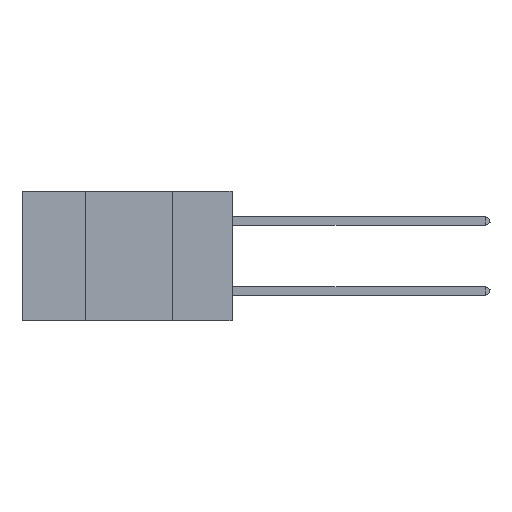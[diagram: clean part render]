
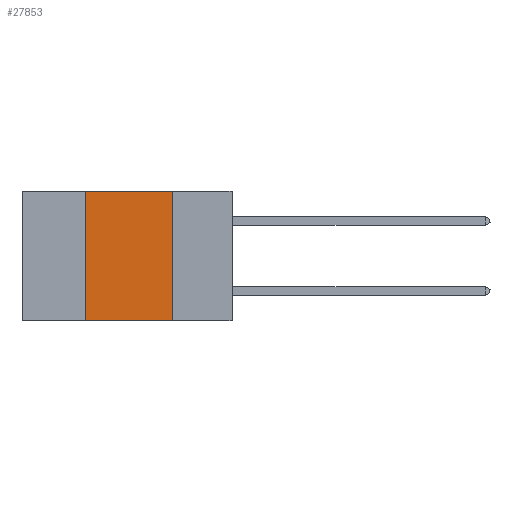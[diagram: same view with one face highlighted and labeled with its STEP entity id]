
A CAD part, left-side view. The second image highlights one B-rep face of the part: STEP entity #27853.
In plain terms, the highlighted planar face has unit normal (-1, 0, 0).
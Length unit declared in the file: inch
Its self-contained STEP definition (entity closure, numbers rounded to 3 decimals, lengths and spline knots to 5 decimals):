
#688 = LINE ( 'NONE', #7129, #45651 ) ;
#830 = DIRECTION ( 'NONE',  ( 0., 0., -1. ) ) ;
#3202 = CARTESIAN_POINT ( 'NONE',  ( 0., 0.6, -0.37 ) ) ;
#3788 = LINE ( 'NONE', #24163, #15774 ) ;
#3945 = DIRECTION ( 'NONE',  ( 0., -1., 0. ) ) ;
#5041 = DIRECTION ( 'NONE',  ( 0., -1., 0. ) ) ;
#7129 = CARTESIAN_POINT ( 'NONE',  ( 0., 0.6, 0. ) ) ;
#8610 = EDGE_CURVE ( 'NONE', #33433, #15304, #44343, .T. ) ;
#11123 = ORIENTED_EDGE ( 'NONE', *, *, #41493, .F. ) ;
#15304 = VERTEX_POINT ( 'NONE', #42648 ) ;
#15774 = VECTOR ( 'NONE', #830, 39.37008 ) ;
#16194 = CARTESIAN_POINT ( 'NONE',  ( 0., 0.6, 0. ) ) ;
#17471 = VECTOR ( 'NONE', #45445, 39.37008 ) ;
#20066 = PLANE ( 'NONE',  #45449 ) ;
#20124 = VERTEX_POINT ( 'NONE', #24308 ) ;
#21398 = DIRECTION ( 'NONE',  ( 0., 0., -1. ) ) ;
#23593 = EDGE_CURVE ( 'NONE', #33433, #20124, #43816, .T. ) ;
#23970 = VERTEX_POINT ( 'NONE', #42732 ) ;
#24080 = DIRECTION ( 'NONE',  ( 1., 0., 0. ) ) ;
#24163 = CARTESIAN_POINT ( 'NONE',  ( 0., 0.17, 0. ) ) ;
#24308 = CARTESIAN_POINT ( 'NONE',  ( 0., 0.42, 0. ) ) ;
#25457 = ORIENTED_EDGE ( 'NONE', *, *, #38529, .F. ) ;
#27853 = ADVANCED_FACE ( 'NONE', ( #35643 ), #20066, .F. ) ;
#33433 = VERTEX_POINT ( 'NONE', #41027 ) ;
#35643 = FACE_OUTER_BOUND ( 'NONE', #48827, .T. ) ;
#38529 = EDGE_CURVE ( 'NONE', #23970, #15304, #3788, .T. ) ;
#38822 = ORIENTED_EDGE ( 'NONE', *, *, #23593, .F. ) ;
#39058 = ORIENTED_EDGE ( 'NONE', *, *, #8610, .T. ) ;
#41027 = CARTESIAN_POINT ( 'NONE',  ( 0., 0.42, -0.37 ) ) ;
#41493 = EDGE_CURVE ( 'NONE', #20124, #23970, #688, .T. ) ;
#42648 = CARTESIAN_POINT ( 'NONE',  ( 0., 0.17, -0.37 ) ) ;
#42732 = CARTESIAN_POINT ( 'NONE',  ( 0., 0.17, 0. ) ) ;
#43760 = VECTOR ( 'NONE', #5041, 39.37008 ) ;
#43816 = LINE ( 'NONE', #45617, #17471 ) ;
#44343 = LINE ( 'NONE', #3202, #43760 ) ;
#45445 = DIRECTION ( 'NONE',  ( 0., 0., 1. ) ) ;
#45449 = AXIS2_PLACEMENT_3D ( 'NONE', #16194, #24080, #21398 ) ;
#45617 = CARTESIAN_POINT ( 'NONE',  ( 0., 0.42, 0. ) ) ;
#45651 = VECTOR ( 'NONE', #3945, 39.37008 ) ;
#48827 = EDGE_LOOP ( 'NONE', ( #25457, #11123, #38822, #39058 ) ) ;
